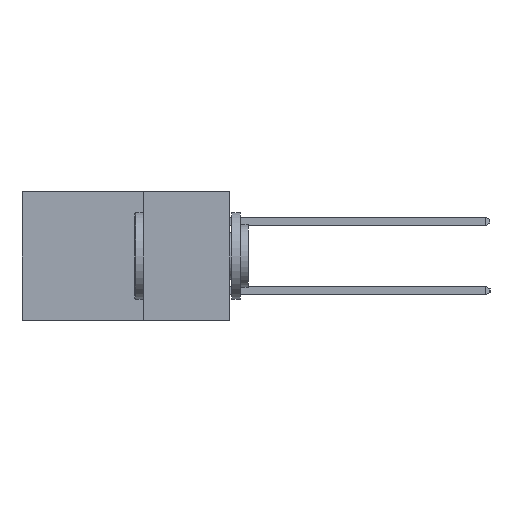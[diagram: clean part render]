
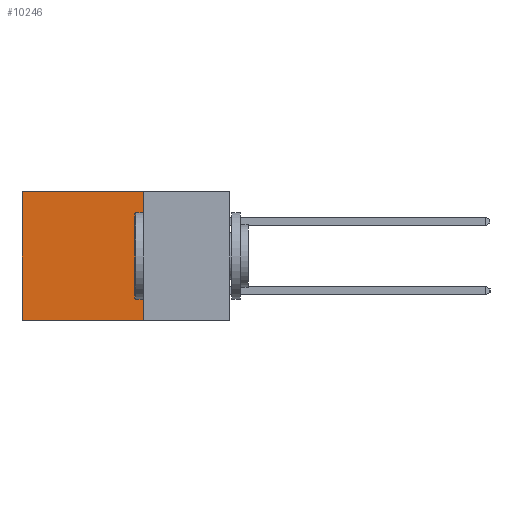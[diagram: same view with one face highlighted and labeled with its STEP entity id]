
A CAD part, left-side view. The second image highlights one B-rep face of the part: STEP entity #10246.
In plain terms, the highlighted planar face has unit normal (-1, 0, 0).
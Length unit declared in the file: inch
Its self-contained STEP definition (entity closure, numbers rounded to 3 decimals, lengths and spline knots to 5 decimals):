
#44 = CARTESIAN_POINT ( 'NONE',  ( 0.2615, 0.25, 0. ) ) ;
#107 = CARTESIAN_POINT ( 'NONE',  ( 0.2615, 0.25, -0.37 ) ) ;
#112 = EDGE_CURVE ( 'NONE', #15101, #18477, #9747, .T. ) ;
#649 = ORIENTED_EDGE ( 'NONE', *, *, #14695, .F. ) ;
#801 = VERTEX_POINT ( 'NONE', #44 ) ;
#1048 = ORIENTED_EDGE ( 'NONE', *, *, #1160, .T. ) ;
#1095 = VERTEX_POINT ( 'NONE', #16377 ) ;
#1160 = EDGE_CURVE ( 'NONE', #801, #15101, #10934, .T. ) ;
#3182 = CARTESIAN_POINT ( 'NONE',  ( 0.2615, 0.6, -0.37 ) ) ;
#4062 = VECTOR ( 'NONE', #18685, 39.37008 ) ;
#4554 = LINE ( 'NONE', #13988, #4062 ) ;
#4976 = PLANE ( 'NONE',  #10558 ) ;
#5226 = VECTOR ( 'NONE', #10251, 39.37008 ) ;
#6615 = DIRECTION ( 'NONE',  ( 0., 0., -1. ) ) ;
#6742 = ORIENTED_EDGE ( 'NONE', *, *, #112, .T. ) ;
#6883 = CARTESIAN_POINT ( 'NONE',  ( 0.2615, 0.25, 0. ) ) ;
#8106 = EDGE_CURVE ( 'NONE', #801, #1095, #13660, .T. ) ;
#8466 = CARTESIAN_POINT ( 'NONE',  ( 0.2615, 0.6, -0.37 ) ) ;
#8748 = VECTOR ( 'NONE', #9779, 39.37008 ) ;
#9747 = LINE ( 'NONE', #3182, #8748 ) ;
#9779 = DIRECTION ( 'NONE',  ( 0., 0., -1. ) ) ;
#10246 = ADVANCED_FACE ( 'NONE', ( #13937 ), #4976, .F. ) ;
#10251 = DIRECTION ( 'NONE',  ( 0., 0., -1. ) ) ;
#10558 = AXIS2_PLACEMENT_3D ( 'NONE', #107, #16014, #6615 ) ;
#10704 = DIRECTION ( 'NONE',  ( 0., 1., 0. ) ) ;
#10934 = LINE ( 'NONE', #6883, #19716 ) ;
#13660 = LINE ( 'NONE', #19605, #5226 ) ;
#13937 = FACE_OUTER_BOUND ( 'NONE', #18318, .T. ) ;
#13988 = CARTESIAN_POINT ( 'NONE',  ( 0.2615, 0.25, -0.37 ) ) ;
#14695 = EDGE_CURVE ( 'NONE', #1095, #18477, #4554, .T. ) ;
#15101 = VERTEX_POINT ( 'NONE', #16615 ) ;
#16014 = DIRECTION ( 'NONE',  ( 1., 0., 0. ) ) ;
#16314 = ORIENTED_EDGE ( 'NONE', *, *, #8106, .F. ) ;
#16377 = CARTESIAN_POINT ( 'NONE',  ( 0.2615, 0.25, -0.37 ) ) ;
#16615 = CARTESIAN_POINT ( 'NONE',  ( 0.2615, 0.6, 0. ) ) ;
#18318 = EDGE_LOOP ( 'NONE', ( #6742, #649, #16314, #1048 ) ) ;
#18477 = VERTEX_POINT ( 'NONE', #8466 ) ;
#18685 = DIRECTION ( 'NONE',  ( 0., 1., 0. ) ) ;
#19605 = CARTESIAN_POINT ( 'NONE',  ( 0.2615, 0.25, -0.37 ) ) ;
#19716 = VECTOR ( 'NONE', #10704, 39.37008 ) ;
